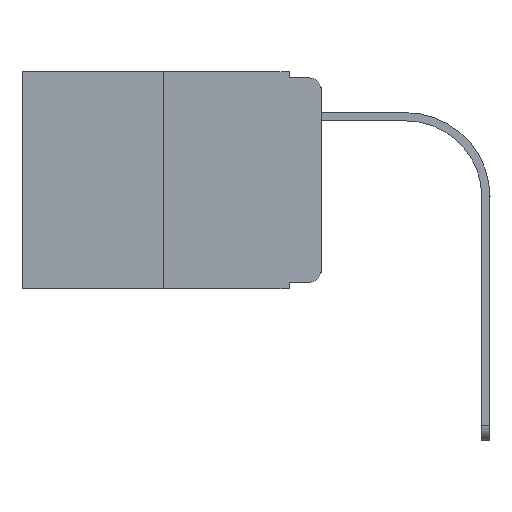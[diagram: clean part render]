
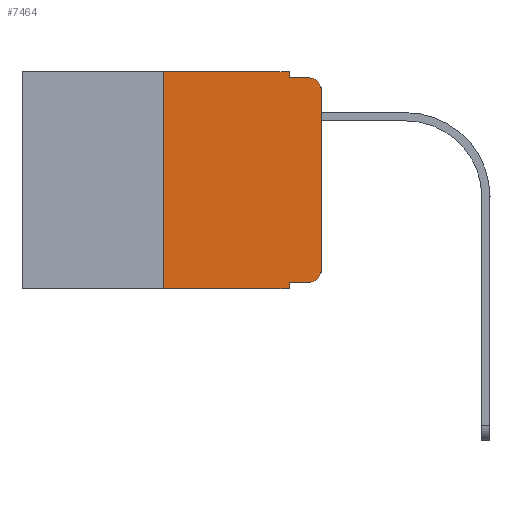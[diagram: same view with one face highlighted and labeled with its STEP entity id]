
A CAD part, left-side view. The second image highlights one B-rep face of the part: STEP entity #7464.
In plain terms, the highlighted planar face has unit normal (-1, 0, 0).
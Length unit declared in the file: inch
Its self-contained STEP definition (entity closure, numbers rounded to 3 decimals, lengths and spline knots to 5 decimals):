
#82 = CARTESIAN_POINT ( 'NONE',  ( 0., 0.25, -0.343 ) ) ;
#188 = LINE ( 'NONE', #1491, #12452 ) ;
#210 = DIRECTION ( 'NONE',  ( 0., 0., -1. ) ) ;
#408 = EDGE_CURVE ( 'NONE', #12031, #3048, #188, .T. ) ;
#448 = VECTOR ( 'NONE', #210, 39.37008 ) ;
#584 = CARTESIAN_POINT ( 'NONE',  ( 0., 0.02, -0.01 ) ) ;
#589 = ORIENTED_EDGE ( 'NONE', *, *, #3361, .T. ) ;
#629 = CARTESIAN_POINT ( 'NONE',  ( 0., 0.051, -0.333 ) ) ;
#639 = VERTEX_POINT ( 'NONE', #9527 ) ;
#1012 = CARTESIAN_POINT ( 'NONE',  ( 0., 0.02, -0.03 ) ) ;
#1311 = ORIENTED_EDGE ( 'NONE', *, *, #9576, .F. ) ;
#1491 = CARTESIAN_POINT ( 'NONE',  ( 0., 0.473, -0.343 ) ) ;
#1990 = CARTESIAN_POINT ( 'NONE',  ( 0., 0.051, -0.333 ) ) ;
#2188 = CARTESIAN_POINT ( 'NONE',  ( 0., 0.051, -0.01 ) ) ;
#2195 = AXIS2_PLACEMENT_3D ( 'NONE', #10735, #8327, #12039 ) ;
#2279 = DIRECTION ( 'NONE',  ( 0., -1., 0. ) ) ;
#2405 = VERTEX_POINT ( 'NONE', #584 ) ;
#2532 = VERTEX_POINT ( 'NONE', #2188 ) ;
#2807 = ORIENTED_EDGE ( 'NONE', *, *, #10229, .T. ) ;
#2885 = DIRECTION ( 'NONE',  ( 0., -1., 0. ) ) ;
#2928 = ORIENTED_EDGE ( 'NONE', *, *, #3021, .T. ) ;
#2958 = LINE ( 'NONE', #7894, #13275 ) ;
#3010 = FACE_OUTER_BOUND ( 'NONE', #12236, .T. ) ;
#3021 = EDGE_CURVE ( 'NONE', #10479, #5049, #5710, .T. ) ;
#3048 = VERTEX_POINT ( 'NONE', #13058 ) ;
#3361 = EDGE_CURVE ( 'NONE', #14411, #4123, #12402, .T. ) ;
#3474 = CARTESIAN_POINT ( 'NONE',  ( 0., 0.02, -0.333 ) ) ;
#3705 = CIRCLE ( 'NONE', #9129, 0.02 ) ;
#3802 = CARTESIAN_POINT ( 'NONE',  ( 0., 0.051, 0. ) ) ;
#4123 = VERTEX_POINT ( 'NONE', #10765 ) ;
#4604 = VECTOR ( 'NONE', #8834, 39.37008 ) ;
#4874 = CARTESIAN_POINT ( 'NONE',  ( 0., 0., 0. ) ) ;
#5049 = VERTEX_POINT ( 'NONE', #3474 ) ;
#5417 = LINE ( 'NONE', #14129, #448 ) ;
#5626 = DIRECTION ( 'NONE',  ( 0., -1., 0. ) ) ;
#5710 = LINE ( 'NONE', #1990, #15491 ) ;
#5759 = CARTESIAN_POINT ( 'NONE',  ( 0., 0.473, 0. ) ) ;
#5791 = VERTEX_POINT ( 'NONE', #12737 ) ;
#6139 = LINE ( 'NONE', #3802, #4604 ) ;
#6252 = ORIENTED_EDGE ( 'NONE', *, *, #6288, .F. ) ;
#6288 = EDGE_CURVE ( 'NONE', #2532, #2405, #11977, .T. ) ;
#6885 = DIRECTION ( 'NONE',  ( 1., 0., 0. ) ) ;
#7018 = EDGE_CURVE ( 'NONE', #5791, #639, #2958, .T. ) ;
#7464 = ADVANCED_FACE ( 'NONE', ( #3010 ), #10608, .F. ) ;
#7623 = AXIS2_PLACEMENT_3D ( 'NONE', #5759, #6885, #11897 ) ;
#7894 = CARTESIAN_POINT ( 'NONE',  ( 0., 0.473, 0. ) ) ;
#8036 = ORIENTED_EDGE ( 'NONE', *, *, #11626, .T. ) ;
#8050 = ORIENTED_EDGE ( 'NONE', *, *, #7018, .F. ) ;
#8287 = EDGE_CURVE ( 'NONE', #639, #2532, #6139, .T. ) ;
#8327 = DIRECTION ( 'NONE',  ( -1., 0., 0. ) ) ;
#8435 = DIRECTION ( 'NONE',  ( -1., 0., 0. ) ) ;
#8447 = ORIENTED_EDGE ( 'NONE', *, *, #8287, .F. ) ;
#8505 = VECTOR ( 'NONE', #9722, 39.37008 ) ;
#8834 = DIRECTION ( 'NONE',  ( 0., 0., -1. ) ) ;
#8843 = DIRECTION ( 'NONE',  ( 0., -1., 0. ) ) ;
#9129 = AXIS2_PLACEMENT_3D ( 'NONE', #1012, #8435, #15712 ) ;
#9527 = CARTESIAN_POINT ( 'NONE',  ( 0., 0.051, 0. ) ) ;
#9576 = EDGE_CURVE ( 'NONE', #10479, #3048, #5417, .T. ) ;
#9722 = DIRECTION ( 'NONE',  ( 0., 0., 1. ) ) ;
#10200 = CIRCLE ( 'NONE', #2195, 0.02 ) ;
#10229 = EDGE_CURVE ( 'NONE', #5049, #14411, #10200, .T. ) ;
#10479 = VERTEX_POINT ( 'NONE', #629 ) ;
#10608 = PLANE ( 'NONE',  #7623 ) ;
#10656 = VECTOR ( 'NONE', #15106, 39.37008 ) ;
#10725 = EDGE_CURVE ( 'NONE', #12031, #5791, #14261, .T. ) ;
#10735 = CARTESIAN_POINT ( 'NONE',  ( 0., 0.02, -0.313 ) ) ;
#10765 = CARTESIAN_POINT ( 'NONE',  ( 0., 0., -0.03 ) ) ;
#11626 = EDGE_CURVE ( 'NONE', #4123, #2405, #3705, .T. ) ;
#11897 = DIRECTION ( 'NONE',  ( 0., 0., -1. ) ) ;
#11977 = LINE ( 'NONE', #12145, #13816 ) ;
#12031 = VERTEX_POINT ( 'NONE', #82 ) ;
#12039 = DIRECTION ( 'NONE',  ( 0., 0., -1. ) ) ;
#12145 = CARTESIAN_POINT ( 'NONE',  ( 0., 0.051, -0.01 ) ) ;
#12236 = EDGE_LOOP ( 'NONE', ( #589, #8036, #6252, #8447, #8050, #12559, #13841, #1311, #2928, #2807 ) ) ;
#12402 = LINE ( 'NONE', #4874, #8505 ) ;
#12452 = VECTOR ( 'NONE', #8843, 39.37008 ) ;
#12559 = ORIENTED_EDGE ( 'NONE', *, *, #10725, .F. ) ;
#12737 = CARTESIAN_POINT ( 'NONE',  ( 0., 0.25, 0. ) ) ;
#13058 = CARTESIAN_POINT ( 'NONE',  ( 0., 0.051, -0.343 ) ) ;
#13104 = CARTESIAN_POINT ( 'NONE',  ( 0., 0., -0.313 ) ) ;
#13275 = VECTOR ( 'NONE', #2885, 39.37008 ) ;
#13816 = VECTOR ( 'NONE', #2279, 39.37008 ) ;
#13841 = ORIENTED_EDGE ( 'NONE', *, *, #408, .T. ) ;
#14129 = CARTESIAN_POINT ( 'NONE',  ( 0., 0.051, 0. ) ) ;
#14176 = CARTESIAN_POINT ( 'NONE',  ( 0., 0.25, 0. ) ) ;
#14261 = LINE ( 'NONE', #14176, #10656 ) ;
#14411 = VERTEX_POINT ( 'NONE', #13104 ) ;
#15106 = DIRECTION ( 'NONE',  ( 0., 0., 1. ) ) ;
#15491 = VECTOR ( 'NONE', #5626, 39.37008 ) ;
#15712 = DIRECTION ( 'NONE',  ( 0., 0., -1. ) ) ;
